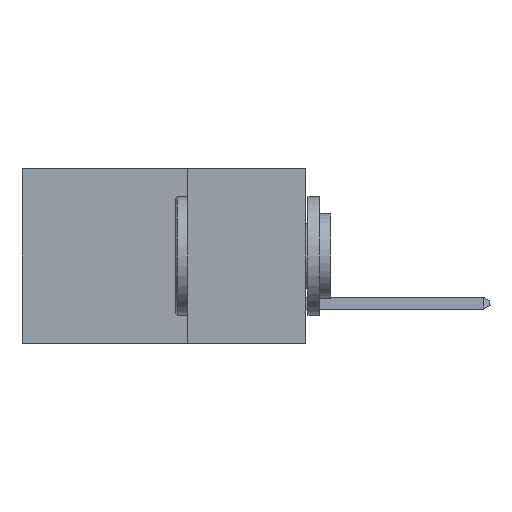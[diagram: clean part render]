
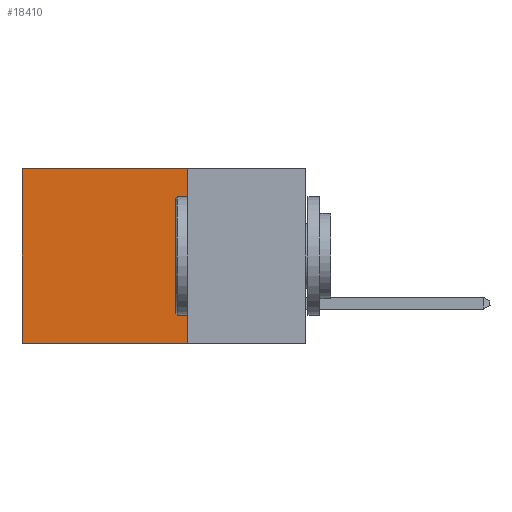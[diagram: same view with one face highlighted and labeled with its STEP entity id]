
A CAD part, left-side view. The second image highlights one B-rep face of the part: STEP entity #18410.
In plain terms, the highlighted planar face has unit normal (-1, 0, 0).
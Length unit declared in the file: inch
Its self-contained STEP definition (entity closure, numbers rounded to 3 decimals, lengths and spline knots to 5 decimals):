
#912 = VERTEX_POINT ( 'NONE', #17163 ) ;
#1873 = CARTESIAN_POINT ( 'NONE',  ( 0.298, 0.25, 0. ) ) ;
#2140 = CARTESIAN_POINT ( 'NONE',  ( 0.298, 0.6, 0. ) ) ;
#3392 = DIRECTION ( 'NONE',  ( 0., 1., 0. ) ) ;
#3406 = EDGE_CURVE ( 'NONE', #912, #9767, #26607, .T. ) ;
#3688 = ORIENTED_EDGE ( 'NONE', *, *, #15107, .T. ) ;
#5466 = EDGE_CURVE ( 'NONE', #24336, #22159, #15177, .T. ) ;
#6265 = CARTESIAN_POINT ( 'NONE',  ( 0.298, 0.25, 0. ) ) ;
#6555 = ORIENTED_EDGE ( 'NONE', *, *, #3406, .F. ) ;
#7320 = VECTOR ( 'NONE', #26153, 39.37008 ) ;
#7823 = ORIENTED_EDGE ( 'NONE', *, *, #15056, .F. ) ;
#8814 = EDGE_LOOP ( 'NONE', ( #18300, #7823, #6555, #3688 ) ) ;
#8853 = FACE_OUTER_BOUND ( 'NONE', #8814, .T. ) ;
#9108 = DIRECTION ( 'NONE',  ( 0., 0., -1. ) ) ;
#9767 = VERTEX_POINT ( 'NONE', #13713 ) ;
#11382 = PLANE ( 'NONE',  #12531 ) ;
#12531 = AXIS2_PLACEMENT_3D ( 'NONE', #23587, #16409, #9108 ) ;
#12562 = VECTOR ( 'NONE', #3392, 39.37008 ) ;
#12888 = CARTESIAN_POINT ( 'NONE',  ( 0.298, 0.6, -0.37 ) ) ;
#13713 = CARTESIAN_POINT ( 'NONE',  ( 0.298, 0.25, -0.37 ) ) ;
#15056 = EDGE_CURVE ( 'NONE', #9767, #22159, #30678, .T. ) ;
#15107 = EDGE_CURVE ( 'NONE', #912, #24336, #23506, .T. ) ;
#15177 = LINE ( 'NONE', #2140, #20861 ) ;
#15446 = CARTESIAN_POINT ( 'NONE',  ( 0.298, 0.25, -0.37 ) ) ;
#16409 = DIRECTION ( 'NONE',  ( 1., 0., 0. ) ) ;
#17163 = CARTESIAN_POINT ( 'NONE',  ( 0.298, 0.25, 0. ) ) ;
#18300 = ORIENTED_EDGE ( 'NONE', *, *, #5466, .T. ) ;
#18410 = ADVANCED_FACE ( 'NONE', ( #8853 ), #11382, .F. ) ;
#20861 = VECTOR ( 'NONE', #26444, 39.37008 ) ;
#22159 = VERTEX_POINT ( 'NONE', #12888 ) ;
#23506 = LINE ( 'NONE', #6265, #29521 ) ;
#23587 = CARTESIAN_POINT ( 'NONE',  ( 0.298, 0.25, 0. ) ) ;
#24336 = VERTEX_POINT ( 'NONE', #29435 ) ;
#25476 = DIRECTION ( 'NONE',  ( 0., 1., 0. ) ) ;
#26153 = DIRECTION ( 'NONE',  ( 0., 0., -1. ) ) ;
#26444 = DIRECTION ( 'NONE',  ( 0., 0., -1. ) ) ;
#26607 = LINE ( 'NONE', #1873, #7320 ) ;
#29435 = CARTESIAN_POINT ( 'NONE',  ( 0.298, 0.6, 0. ) ) ;
#29521 = VECTOR ( 'NONE', #25476, 39.37008 ) ;
#30678 = LINE ( 'NONE', #15446, #12562 ) ;
